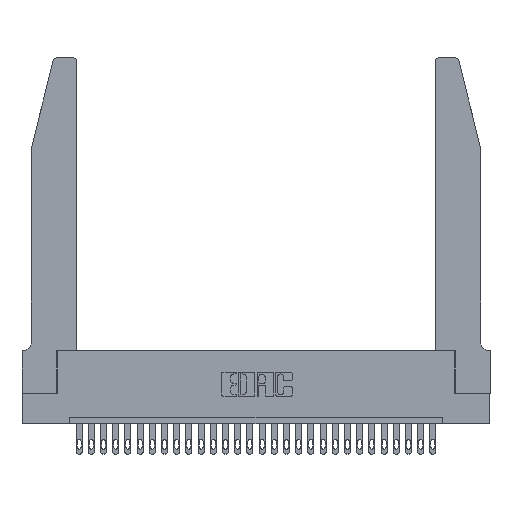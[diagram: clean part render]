
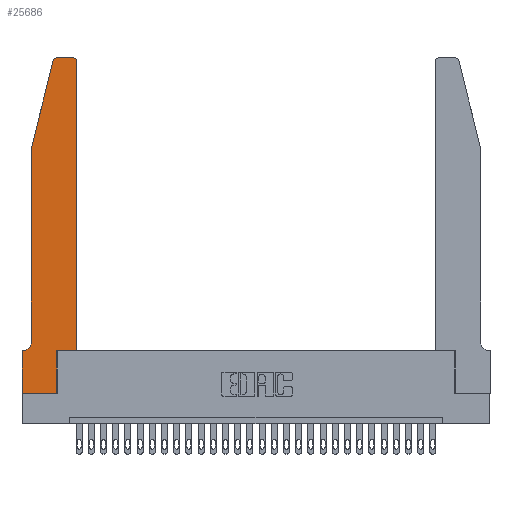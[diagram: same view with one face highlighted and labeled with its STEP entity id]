
A CAD part, top view. The second image highlights one B-rep face of the part: STEP entity #25686.
In plain terms, the highlighted planar face has unit normal (0, 0, 1).
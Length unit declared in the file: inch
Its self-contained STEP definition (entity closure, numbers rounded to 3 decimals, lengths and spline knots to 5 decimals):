
#389 = VECTOR ( 'NONE', #21255, 39.37008 ) ;
#575 = VERTEX_POINT ( 'NONE', #27916 ) ;
#928 = FACE_OUTER_BOUND ( 'NONE', #25162, .T. ) ;
#1032 = VERTEX_POINT ( 'NONE', #7294 ) ;
#1565 = ORIENTED_EDGE ( 'NONE', *, *, #10731, .T. ) ;
#1580 = VECTOR ( 'NONE', #3534, 39.37008 ) ;
#1588 = DIRECTION ( 'NONE',  ( -0.239, -0.971, 0. ) ) ;
#1591 = DIRECTION ( 'NONE',  ( 0., 0., 1. ) ) ;
#1948 = DIRECTION ( 'NONE',  ( 0., 0., 1. ) ) ;
#2073 = DIRECTION ( 'NONE',  ( 0., 1., 0. ) ) ;
#2503 = VECTOR ( 'NONE', #10674, 39.37008 ) ;
#2550 = DIRECTION ( 'NONE',  ( 0., 0., 1. ) ) ;
#2619 = CARTESIAN_POINT ( 'NONE',  ( 0.0755, 2., 0.37 ) ) ;
#2733 = VERTEX_POINT ( 'NONE', #26808 ) ;
#2878 = VERTEX_POINT ( 'NONE', #24361 ) ;
#3094 = EDGE_CURVE ( 'NONE', #4589, #12039, #14107, .T. ) ;
#3312 = CIRCLE ( 'NONE', #21448, 0.03 ) ;
#3395 = CARTESIAN_POINT ( 'NONE',  ( 0., 0., 0.37 ) ) ;
#3417 = CARTESIAN_POINT ( 'NONE',  ( 0., 0., 0.37 ) ) ;
#3534 = DIRECTION ( 'NONE',  ( -1., 0., 0. ) ) ;
#3697 = CARTESIAN_POINT ( 'NONE',  ( 0., 0.35, 0.37 ) ) ;
#3859 = LINE ( 'NONE', #27560, #11827 ) ;
#4006 = DIRECTION ( 'NONE',  ( 1., 0., 0. ) ) ;
#4134 = AXIS2_PLACEMENT_3D ( 'NONE', #14642, #1591, #12379 ) ;
#4408 = LINE ( 'NONE', #26205, #27419 ) ;
#4589 = VERTEX_POINT ( 'NONE', #17806 ) ;
#4608 = ORIENTED_EDGE ( 'NONE', *, *, #20418, .T. ) ;
#4620 = ORIENTED_EDGE ( 'NONE', *, *, #3094, .T. ) ;
#5134 = EDGE_CURVE ( 'NONE', #10868, #4589, #13445, .T. ) ;
#5237 = VECTOR ( 'NONE', #9399, 39.37008 ) ;
#5824 = EDGE_CURVE ( 'NONE', #12068, #2878, #4408, .T. ) ;
#7294 = CARTESIAN_POINT ( 'NONE',  ( 0., 0., 0.37 ) ) ;
#7569 = DIRECTION ( 'NONE',  ( 0., -1., 0. ) ) ;
#7576 = CIRCLE ( 'NONE', #9653, 0.03 ) ;
#7621 = EDGE_CURVE ( 'NONE', #1032, #12068, #25572, .T. ) ;
#7828 = DIRECTION ( 'NONE',  ( -1., 0., 0. ) ) ;
#7997 = CARTESIAN_POINT ( 'NONE',  ( 0.4205, 2.75, 0.37 ) ) ;
#8179 = AXIS2_PLACEMENT_3D ( 'NONE', #8966, #16080, #11650 ) ;
#8302 = LINE ( 'NONE', #3417, #28899 ) ;
#8403 = CARTESIAN_POINT ( 'NONE',  ( 0.4505, 0.35, 0.37 ) ) ;
#8966 = CARTESIAN_POINT ( 'NONE',  ( 0.0055, 0.42, 0.37 ) ) ;
#9006 = EDGE_CURVE ( 'NONE', #28788, #10868, #11141, .T. ) ;
#9399 = DIRECTION ( 'NONE',  ( 0., -1., 0. ) ) ;
#9653 = AXIS2_PLACEMENT_3D ( 'NONE', #26771, #2550, #11212 ) ;
#10190 = VERTEX_POINT ( 'NONE', #12664 ) ;
#10483 = CARTESIAN_POINT ( 'NONE',  ( 0.284, 2.72, 0.37 ) ) ;
#10674 = DIRECTION ( 'NONE',  ( 1., 0., 0. ) ) ;
#10731 = EDGE_CURVE ( 'NONE', #575, #2733, #11271, .T. ) ;
#10868 = VERTEX_POINT ( 'NONE', #25176 ) ;
#10914 = VECTOR ( 'NONE', #2073, 39.37008 ) ;
#11141 = LINE ( 'NONE', #2619, #5237 ) ;
#11212 = DIRECTION ( 'NONE',  ( 1., 0., 0. ) ) ;
#11271 = LINE ( 'NONE', #8403, #10914 ) ;
#11518 = ORIENTED_EDGE ( 'NONE', *, *, #28593, .T. ) ;
#11650 = DIRECTION ( 'NONE',  ( -1., 0., 0. ) ) ;
#11827 = VECTOR ( 'NONE', #7828, 39.37008 ) ;
#12039 = VERTEX_POINT ( 'NONE', #3697 ) ;
#12068 = VERTEX_POINT ( 'NONE', #25442 ) ;
#12112 = CARTESIAN_POINT ( 'NONE',  ( 0.0755, 2., 0.37 ) ) ;
#12379 = DIRECTION ( 'NONE',  ( 1., 0., 0. ) ) ;
#12664 = CARTESIAN_POINT ( 'NONE',  ( 0.284, 2.75, 0.37 ) ) ;
#13024 = ORIENTED_EDGE ( 'NONE', *, *, #9006, .T. ) ;
#13367 = EDGE_CURVE ( 'NONE', #10190, #24392, #3312, .T. ) ;
#13445 = CIRCLE ( 'NONE', #8179, 0.07 ) ;
#14107 = LINE ( 'NONE', #22964, #1580 ) ;
#14642 = CARTESIAN_POINT ( 'NONE',  ( 0., 0.35, 0.37 ) ) ;
#14835 = EDGE_CURVE ( 'NONE', #2878, #575, #19982, .T. ) ;
#16080 = DIRECTION ( 'NONE',  ( 0., 0., -1. ) ) ;
#16088 = LINE ( 'NONE', #28276, #23487 ) ;
#17022 = ORIENTED_EDGE ( 'NONE', *, *, #5134, .T. ) ;
#17038 = DIRECTION ( 'NONE',  ( 0., 1., 0. ) ) ;
#17058 = EDGE_CURVE ( 'NONE', #2733, #22852, #7576, .T. ) ;
#17575 = ORIENTED_EDGE ( 'NONE', *, *, #14835, .T. ) ;
#17806 = CARTESIAN_POINT ( 'NONE',  ( 0.0055, 0.35, 0.37 ) ) ;
#19982 = LINE ( 'NONE', #23760, #2503 ) ;
#20418 = EDGE_CURVE ( 'NONE', #22852, #10190, #3859, .T. ) ;
#20734 = ORIENTED_EDGE ( 'NONE', *, *, #7621, .T. ) ;
#20890 = CARTESIAN_POINT ( 'NONE',  ( 0.25487, 2.72718, 0.37 ) ) ;
#21161 = ORIENTED_EDGE ( 'NONE', *, *, #5824, .T. ) ;
#21255 = DIRECTION ( 'NONE',  ( 1., 0., 0. ) ) ;
#21448 = AXIS2_PLACEMENT_3D ( 'NONE', #10483, #1948, #4006 ) ;
#21686 = EDGE_CURVE ( 'NONE', #12039, #1032, #8302, .T. ) ;
#22095 = ORIENTED_EDGE ( 'NONE', *, *, #17058, .T. ) ;
#22852 = VERTEX_POINT ( 'NONE', #7997 ) ;
#22964 = CARTESIAN_POINT ( 'NONE',  ( 0.0755, 0.35, 0.37 ) ) ;
#23487 = VECTOR ( 'NONE', #1588, 39.37008 ) ;
#23760 = CARTESIAN_POINT ( 'NONE',  ( 0.4505, 0.35, 0.37 ) ) ;
#24361 = CARTESIAN_POINT ( 'NONE',  ( 0.2865, 0.35, 0.37 ) ) ;
#24392 = VERTEX_POINT ( 'NONE', #20890 ) ;
#25162 = EDGE_LOOP ( 'NONE', ( #4608, #27728, #11518, #13024, #17022, #4620, #26945, #20734, #21161, #17575, #1565, #22095 ) ) ;
#25176 = CARTESIAN_POINT ( 'NONE',  ( 0.0755, 0.42, 0.37 ) ) ;
#25442 = CARTESIAN_POINT ( 'NONE',  ( 0.2865, 0., 0.37 ) ) ;
#25572 = LINE ( 'NONE', #3395, #389 ) ;
#25686 = ADVANCED_FACE ( 'NONE', ( #928 ), #27613, .T. ) ;
#26205 = CARTESIAN_POINT ( 'NONE',  ( 0.2865, 0.35, 0.37 ) ) ;
#26771 = CARTESIAN_POINT ( 'NONE',  ( 0.4205, 2.72, 0.37 ) ) ;
#26808 = CARTESIAN_POINT ( 'NONE',  ( 0.4505, 2.72, 0.37 ) ) ;
#26945 = ORIENTED_EDGE ( 'NONE', *, *, #21686, .T. ) ;
#27419 = VECTOR ( 'NONE', #17038, 39.37008 ) ;
#27560 = CARTESIAN_POINT ( 'NONE',  ( 0.2605, 2.75, 0.37 ) ) ;
#27613 = PLANE ( 'NONE',  #4134 ) ;
#27728 = ORIENTED_EDGE ( 'NONE', *, *, #13367, .T. ) ;
#27916 = CARTESIAN_POINT ( 'NONE',  ( 0.4505, 0.35, 0.37 ) ) ;
#28276 = CARTESIAN_POINT ( 'NONE',  ( 0.0755, 2., 0.37 ) ) ;
#28593 = EDGE_CURVE ( 'NONE', #24392, #28788, #16088, .T. ) ;
#28788 = VERTEX_POINT ( 'NONE', #12112 ) ;
#28899 = VECTOR ( 'NONE', #7569, 39.37008 ) ;
